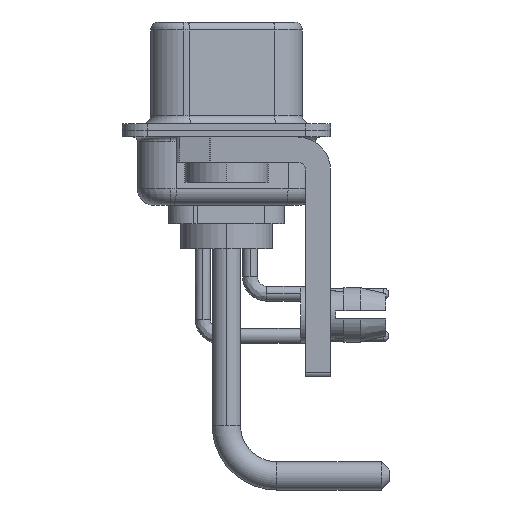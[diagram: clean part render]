
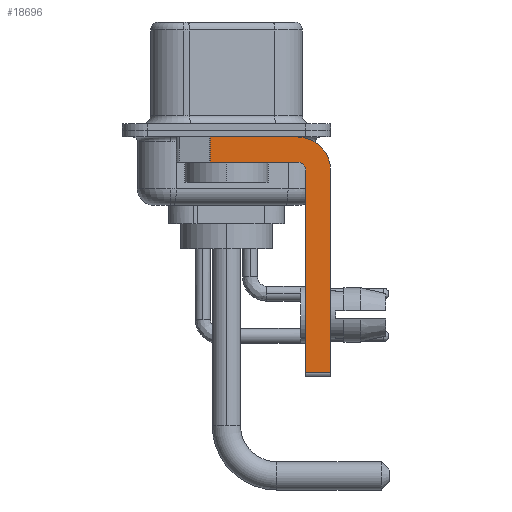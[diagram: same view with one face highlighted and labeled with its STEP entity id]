
A CAD part, left-side view. The second image highlights one B-rep face of the part: STEP entity #18696.
In plain terms, the highlighted planar face has unit normal (-1, 0, 0).
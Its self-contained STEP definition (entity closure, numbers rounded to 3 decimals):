
#137 = DIRECTION ( 'NONE',  ( 0., 0., 1. ) ) ;
#455 = AXIS2_PLACEMENT_3D ( 'NONE', #14543, #28110, #25404 ) ;
#1142 = CARTESIAN_POINT ( 'NONE',  ( -2.9, -6.25, -14.55 ) ) ;
#1431 = EDGE_CURVE ( 'NONE', #28164, #26222, #21807, .T. ) ;
#2546 = EDGE_CURVE ( 'NONE', #9167, #19254, #20927, .T. ) ;
#2730 = CARTESIAN_POINT ( 'NONE',  ( -2.9, -4.75, -2.4 ) ) ;
#3601 = EDGE_CURVE ( 'NONE', #14768, #9167, #19452, .T. ) ;
#3629 = CARTESIAN_POINT ( 'NONE',  ( -2.9, -4.25, -1.9 ) ) ;
#3635 = CIRCLE ( 'NONE', #5901, 0.5 ) ;
#4037 = ORIENTED_EDGE ( 'NONE', *, *, #2546, .F. ) ;
#4577 = EDGE_CURVE ( 'NONE', #28164, #23106, #24921, .T. ) ;
#4608 = FACE_OUTER_BOUND ( 'NONE', #14629, .T. ) ;
#5136 = CARTESIAN_POINT ( 'NONE',  ( -2.9, 0.978, -1.9 ) ) ;
#5317 = DIRECTION ( 'NONE',  ( -1., 0., 0. ) ) ;
#5611 = CARTESIAN_POINT ( 'NONE',  ( -2.9, -4.25, -0.4 ) ) ;
#5613 = DIRECTION ( 'NONE',  ( 0., 1., 0. ) ) ;
#5656 = ORIENTED_EDGE ( 'NONE', *, *, #20528, .T. ) ;
#5901 = AXIS2_PLACEMENT_3D ( 'NONE', #18555, #5317, #20566 ) ;
#6340 = DIRECTION ( 'NONE',  ( 0., -1., 0. ) ) ;
#6546 = ORIENTED_EDGE ( 'NONE', *, *, #23986, .F. ) ;
#6937 = CARTESIAN_POINT ( 'NONE',  ( -2.9, -4.75, -14.55 ) ) ;
#7682 = DIRECTION ( 'NONE',  ( 0., 0., -1. ) ) ;
#9167 = VERTEX_POINT ( 'NONE', #5611 ) ;
#9699 = LINE ( 'NONE', #5136, #23978 ) ;
#10067 = EDGE_CURVE ( 'NONE', #26222, #12220, #3635, .T. ) ;
#10547 = CARTESIAN_POINT ( 'NONE',  ( -2.9, 0.978, -1.9 ) ) ;
#11013 = PLANE ( 'NONE',  #26232 ) ;
#11590 = CARTESIAN_POINT ( 'NONE',  ( -2.9, -4.25, -2.4 ) ) ;
#11683 = CARTESIAN_POINT ( 'NONE',  ( -2.9, -4.25, -1.9 ) ) ;
#12220 = VERTEX_POINT ( 'NONE', #11683 ) ;
#13546 = EDGE_CURVE ( 'NONE', #19254, #23106, #26959, .T. ) ;
#14543 = CARTESIAN_POINT ( 'NONE',  ( -2.9, -4.25, -2.4 ) ) ;
#14629 = EDGE_LOOP ( 'NONE', ( #22903, #5656, #6546, #15784, #17197, #27793, #18059, #4037 ) ) ;
#14768 = VERTEX_POINT ( 'NONE', #23681 ) ;
#14774 = VERTEX_POINT ( 'NONE', #10547 ) ;
#15784 = ORIENTED_EDGE ( 'NONE', *, *, #10067, .F. ) ;
#15997 = VECTOR ( 'NONE', #7682, 1000. ) ;
#16421 = LINE ( 'NONE', #3629, #26489 ) ;
#17197 = ORIENTED_EDGE ( 'NONE', *, *, #1431, .F. ) ;
#17776 = VECTOR ( 'NONE', #6340, 1000. ) ;
#18059 = ORIENTED_EDGE ( 'NONE', *, *, #13546, .F. ) ;
#18090 = CARTESIAN_POINT ( 'NONE',  ( -2.9, -6.25, -2.4 ) ) ;
#18555 = CARTESIAN_POINT ( 'NONE',  ( -2.9, -4.25, -2.4 ) ) ;
#18696 = ADVANCED_FACE ( 'NONE', ( #4608 ), #11013, .F. ) ;
#19254 = VERTEX_POINT ( 'NONE', #18090 ) ;
#19452 = LINE ( 'NONE', #26178, #17776 ) ;
#19992 = DIRECTION ( 'NONE',  ( 0., 0., -1. ) ) ;
#20528 = EDGE_CURVE ( 'NONE', #14768, #14774, #9699, .T. ) ;
#20566 = DIRECTION ( 'NONE',  ( 0., 0., 1. ) ) ;
#20927 = CIRCLE ( 'NONE', #455, 2. ) ;
#20946 = VECTOR ( 'NONE', #137, 1000. ) ;
#21807 = LINE ( 'NONE', #24236, #20946 ) ;
#22647 = DIRECTION ( 'NONE',  ( 0., -1., 0. ) ) ;
#22903 = ORIENTED_EDGE ( 'NONE', *, *, #3601, .F. ) ;
#23106 = VERTEX_POINT ( 'NONE', #1142 ) ;
#23681 = CARTESIAN_POINT ( 'NONE',  ( -2.9, 0.978, -0.4 ) ) ;
#23978 = VECTOR ( 'NONE', #25102, 1000. ) ;
#23986 = EDGE_CURVE ( 'NONE', #12220, #14774, #16421, .T. ) ;
#24236 = CARTESIAN_POINT ( 'NONE',  ( -2.9, -4.75, -14.8 ) ) ;
#24270 = VECTOR ( 'NONE', #22647, 1000. ) ;
#24921 = LINE ( 'NONE', #25196, #24270 ) ;
#25102 = DIRECTION ( 'NONE',  ( 0., 0., -1. ) ) ;
#25196 = CARTESIAN_POINT ( 'NONE',  ( -2.9, -4.25, -14.55 ) ) ;
#25404 = DIRECTION ( 'NONE',  ( 0., 0., -1. ) ) ;
#26178 = CARTESIAN_POINT ( 'NONE',  ( -2.9, 3., -0.4 ) ) ;
#26222 = VERTEX_POINT ( 'NONE', #2730 ) ;
#26232 = AXIS2_PLACEMENT_3D ( 'NONE', #11590, #26427, #19992 ) ;
#26427 = DIRECTION ( 'NONE',  ( 1., 0., 0. ) ) ;
#26489 = VECTOR ( 'NONE', #5613, 1000. ) ;
#26959 = LINE ( 'NONE', #27239, #15997 ) ;
#27239 = CARTESIAN_POINT ( 'NONE',  ( -2.9, -6.25, -2.4 ) ) ;
#27793 = ORIENTED_EDGE ( 'NONE', *, *, #4577, .T. ) ;
#28110 = DIRECTION ( 'NONE',  ( 1., 0., 0. ) ) ;
#28164 = VERTEX_POINT ( 'NONE', #6937 ) ;
